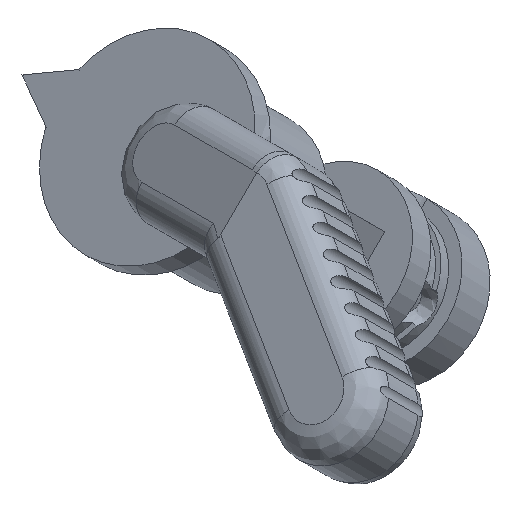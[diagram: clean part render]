
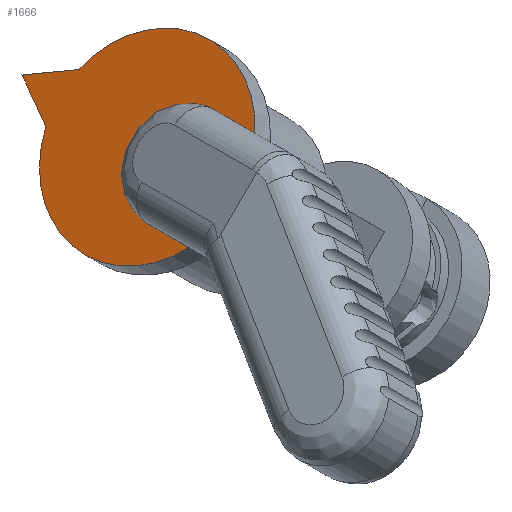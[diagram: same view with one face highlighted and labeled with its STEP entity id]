
A CAD part, isometric view. The second image highlights one B-rep face of the part: STEP entity #1666.
In plain terms, the highlighted planar face has unit normal (-0.707, 0, 0.707).
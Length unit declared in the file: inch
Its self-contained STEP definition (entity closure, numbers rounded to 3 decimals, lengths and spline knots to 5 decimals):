
#182=CIRCLE('',#1798,0.125);
#193=CIRCLE('',#1828,0.23622);
#194=CIRCLE('',#1830,0.23622);
#287=FACE_OUTER_BOUND('',#381,.T.);
#381=EDGE_LOOP('',(#1472,#1473,#1474,#1475,#1476,#1477,#1478));
#465=LINE('',#3036,#583);
#482=LINE('',#3206,#600);
#503=LINE('',#3869,#621);
#505=LINE('',#3873,#623);
#583=VECTOR('',#2053,0.3937);
#600=VECTOR('',#2132,0.3937);
#621=VECTOR('',#2213,0.3937);
#623=VECTOR('',#2217,0.3937);
#736=VERTEX_POINT('',#3016);
#739=VERTEX_POINT('',#3025);
#763=VERTEX_POINT('',#3203);
#764=VERTEX_POINT('',#3205);
#797=VERTEX_POINT('',#3866);
#798=VERTEX_POINT('',#3868);
#799=VERTEX_POINT('',#3872);
#935=EDGE_CURVE('',#739,#736,#465,.F.);
#974=EDGE_CURVE('',#764,#763,#482,.T.);
#978=EDGE_CURVE('',#763,#736,#182,.T.);
#1030=EDGE_CURVE('',#798,#797,#503,.T.);
#1032=EDGE_CURVE('',#799,#798,#505,.T.);
#1034=EDGE_CURVE('',#799,#739,#193,.T.);
#1035=EDGE_CURVE('',#797,#764,#194,.T.);
#1472=ORIENTED_EDGE('',*,*,#1035,.T.);
#1473=ORIENTED_EDGE('',*,*,#974,.T.);
#1474=ORIENTED_EDGE('',*,*,#978,.T.);
#1475=ORIENTED_EDGE('',*,*,#935,.F.);
#1476=ORIENTED_EDGE('',*,*,#1034,.F.);
#1477=ORIENTED_EDGE('',*,*,#1032,.T.);
#1478=ORIENTED_EDGE('',*,*,#1030,.T.);
#1579=PLANE('',#1831);
#1666=ADVANCED_FACE('',(#287),#1579,.T.);
#1798=AXIS2_PLACEMENT_3D('',#3212,#2140,#2141);
#1828=AXIS2_PLACEMENT_3D('',#3876,#2221,#2222);
#1830=AXIS2_PLACEMENT_3D('',#3878,#2225,#2226);
#1831=AXIS2_PLACEMENT_3D('',#3879,#2227,#2228);
#2053=DIRECTION('',(0.,-1.,0.));
#2132=DIRECTION('',(0.,1.,0.));
#2140=DIRECTION('center_axis',(0.707,0.,-0.707));
#2141=DIRECTION('ref_axis',(-0.707,0.,-0.707));
#2213=DIRECTION('',(-0.354,-0.866,-0.354));
#2217=DIRECTION('',(-0.354,0.866,-0.354));
#2221=DIRECTION('center_axis',(0.707,0.,-0.707));
#2222=DIRECTION('ref_axis',(0.,-1.,0.));
#2225=DIRECTION('center_axis',(-0.707,0.,0.707));
#2226=DIRECTION('ref_axis',(0.,-1.,0.));
#2227=DIRECTION('center_axis',(-0.707,0.,0.707));
#2228=DIRECTION('ref_axis',(0.,-1.,0.));
#3016=CARTESIAN_POINT('',(0.05793,-0.12013,0.25257));
#3025=CARTESIAN_POINT('',(0.05793,-0.2005,0.25257));
#3036=CARTESIAN_POINT('',(0.05793,-0.15355,0.25257));
#3203=CARTESIAN_POINT('',(-0.11878,-0.125,0.07586));
#3205=CARTESIAN_POINT('',(-0.11878,-0.20044,0.07586));
#3206=CARTESIAN_POINT('',(-0.11878,-0.725,0.07586));
#3212=CARTESIAN_POINT('Origin',(-0.03039,-0.125,0.16425));
#3866=CARTESIAN_POINT('',(-0.07467,0.22777,0.11997));
#3868=CARTESIAN_POINT('',(-0.03039,0.33622,0.16425));
#3869=CARTESIAN_POINT('',(-0.03039,0.33622,0.16425));
#3872=CARTESIAN_POINT('',(0.01388,0.22777,0.20852));
#3873=CARTESIAN_POINT('',(0.01388,0.22777,0.20852));
#3876=CARTESIAN_POINT('Origin',(-0.03039,0.,0.16425));
#3878=CARTESIAN_POINT('Origin',(-0.03039,0.,0.16425));
#3879=CARTESIAN_POINT('Origin',(-0.03039,0.06789,
0.16425));
